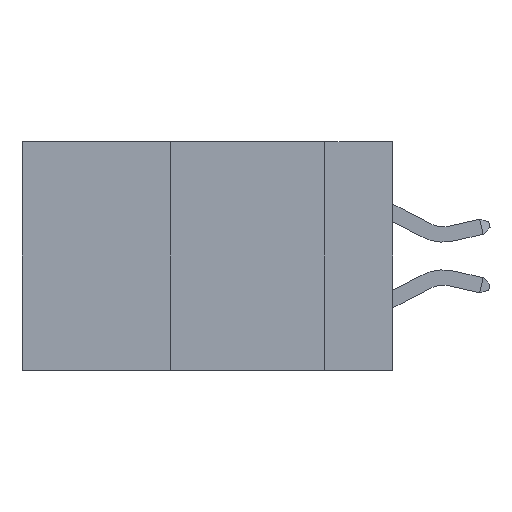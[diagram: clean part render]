
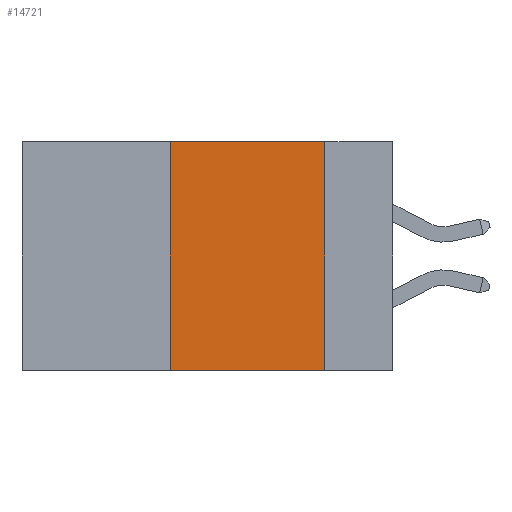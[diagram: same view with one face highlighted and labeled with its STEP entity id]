
A CAD part, left-side view. The second image highlights one B-rep face of the part: STEP entity #14721.
In plain terms, the highlighted planar face has unit normal (-1, 0, 0).
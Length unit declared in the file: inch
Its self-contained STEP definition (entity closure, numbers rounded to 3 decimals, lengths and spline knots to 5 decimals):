
#60 = LINE ( 'NONE', #8559, #19582 ) ;
#1080 = EDGE_CURVE ( 'NONE', #13899, #19810, #6628, .T. ) ;
#1740 = VECTOR ( 'NONE', #20913, 39.37008 ) ;
#2148 = LINE ( 'NONE', #10227, #1740 ) ;
#3196 = ORIENTED_EDGE ( 'NONE', *, *, #5862, .F. ) ;
#3532 = CARTESIAN_POINT ( 'NONE',  ( 0., 0.36, 0. ) ) ;
#3990 = VECTOR ( 'NONE', #11871, 39.37008 ) ;
#4148 = DIRECTION ( 'NONE',  ( 0., 0., -1. ) ) ;
#4818 = CARTESIAN_POINT ( 'NONE',  ( 0., 0.6, -0.37 ) ) ;
#5009 = ORIENTED_EDGE ( 'NONE', *, *, #8620, .F. ) ;
#5039 = VERTEX_POINT ( 'NONE', #3532 ) ;
#5862 = EDGE_CURVE ( 'NONE', #5039, #9765, #6717, .T. ) ;
#6124 = CARTESIAN_POINT ( 'NONE',  ( 0., 0.36, -0.37 ) ) ;
#6628 = LINE ( 'NONE', #4818, #3990 ) ;
#6717 = LINE ( 'NONE', #11862, #17635 ) ;
#8559 = CARTESIAN_POINT ( 'NONE',  ( 0., 0.11, 0. ) ) ;
#8564 = EDGE_CURVE ( 'NONE', #9765, #19810, #60, .T. ) ;
#8620 = EDGE_CURVE ( 'NONE', #13899, #5039, #2148, .T. ) ;
#8911 = EDGE_LOOP ( 'NONE', ( #11718, #3196, #5009, #17305 ) ) ;
#9256 = DIRECTION ( 'NONE',  ( 1., 0., 0. ) ) ;
#9636 = CARTESIAN_POINT ( 'NONE',  ( 0., 0.11, -0.37 ) ) ;
#9765 = VERTEX_POINT ( 'NONE', #14270 ) ;
#10227 = CARTESIAN_POINT ( 'NONE',  ( 0., 0.36, 0. ) ) ;
#11718 = ORIENTED_EDGE ( 'NONE', *, *, #8564, .F. ) ;
#11862 = CARTESIAN_POINT ( 'NONE',  ( 0., 0.6, 0. ) ) ;
#11871 = DIRECTION ( 'NONE',  ( 0., -1., 0. ) ) ;
#12637 = AXIS2_PLACEMENT_3D ( 'NONE', #20873, #9256, #17513 ) ;
#13899 = VERTEX_POINT ( 'NONE', #6124 ) ;
#14164 = FACE_OUTER_BOUND ( 'NONE', #8911, .T. ) ;
#14270 = CARTESIAN_POINT ( 'NONE',  ( 0., 0.11, 0. ) ) ;
#14721 = ADVANCED_FACE ( 'NONE', ( #14164 ), #15947, .F. ) ;
#15947 = PLANE ( 'NONE',  #12637 ) ;
#17305 = ORIENTED_EDGE ( 'NONE', *, *, #1080, .T. ) ;
#17513 = DIRECTION ( 'NONE',  ( 0., 0., -1. ) ) ;
#17635 = VECTOR ( 'NONE', #18673, 39.37008 ) ;
#18673 = DIRECTION ( 'NONE',  ( 0., -1., 0. ) ) ;
#19582 = VECTOR ( 'NONE', #4148, 39.37008 ) ;
#19810 = VERTEX_POINT ( 'NONE', #9636 ) ;
#20873 = CARTESIAN_POINT ( 'NONE',  ( 0., 0.6, 0. ) ) ;
#20913 = DIRECTION ( 'NONE',  ( 0., 0., 1. ) ) ;
